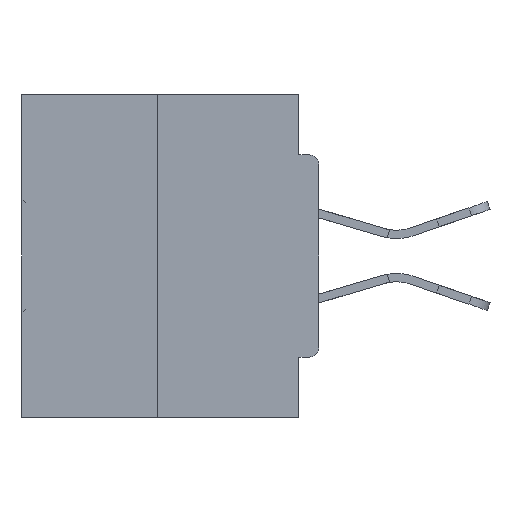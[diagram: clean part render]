
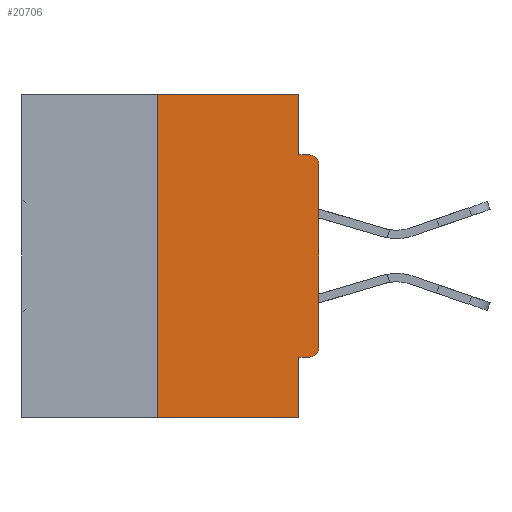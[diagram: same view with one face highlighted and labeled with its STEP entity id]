
A CAD part, left-side view. The second image highlights one B-rep face of the part: STEP entity #20706.
In plain terms, the highlighted planar face has unit normal (-1, 0, 0).
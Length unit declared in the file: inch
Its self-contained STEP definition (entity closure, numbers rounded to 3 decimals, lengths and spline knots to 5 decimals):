
#2132 = CARTESIAN_POINT ( 'NONE',  ( 0., 0.015, -0.3915 ) ) ;
#3215 = ORIENTED_EDGE ( 'NONE', *, *, #10793, .F. ) ;
#3458 = AXIS2_PLACEMENT_3D ( 'NONE', #44078, #10259, #24058 ) ;
#3764 = LINE ( 'NONE', #19741, #40577 ) ;
#4385 = VECTOR ( 'NONE', #37120, 39.37008 ) ;
#5141 = LINE ( 'NONE', #14139, #30230 ) ;
#6019 = EDGE_LOOP ( 'NONE', ( #20802, #9679, #41774, #3215, #23538, #33979, #34503, #25848, #26507, #16166 ) ) ;
#6390 = CARTESIAN_POINT ( 'NONE',  ( 0., 0.25, 0. ) ) ;
#6479 = CARTESIAN_POINT ( 'NONE',  ( 0., 0.015, -0.4065 ) ) ;
#6637 = CARTESIAN_POINT ( 'NONE',  ( 0., 0., 0. ) ) ;
#6655 = PLANE ( 'NONE',  #3458 ) ;
#8766 = EDGE_CURVE ( 'NONE', #9557, #28102, #12929, .T. ) ;
#9229 = EDGE_CURVE ( 'NONE', #41579, #10682, #3764, .T. ) ;
#9557 = VERTEX_POINT ( 'NONE', #23815 ) ;
#9679 = ORIENTED_EDGE ( 'NONE', *, *, #15289, .F. ) ;
#9711 = DIRECTION ( 'NONE',  ( 0., -1., 0. ) ) ;
#10259 = DIRECTION ( 'NONE',  ( 1., 0., 0. ) ) ;
#10342 = VERTEX_POINT ( 'NONE', #38092 ) ;
#10682 = VERTEX_POINT ( 'NONE', #34800 ) ;
#10779 = CARTESIAN_POINT ( 'NONE',  ( 0., 0.46, 0. ) ) ;
#10793 = EDGE_CURVE ( 'NONE', #10682, #10342, #41548, .T. ) ;
#11541 = CARTESIAN_POINT ( 'NONE',  ( 0., 0., -0.3915 ) ) ;
#12639 = DIRECTION ( 'NONE',  ( -1., 0., 0. ) ) ;
#12929 = LINE ( 'NONE', #37290, #25717 ) ;
#13161 = CARTESIAN_POINT ( 'NONE',  ( 0., 0.015, -0.1085 ) ) ;
#13564 = DIRECTION ( 'NONE',  ( 0., 0., 1. ) ) ;
#14139 = CARTESIAN_POINT ( 'NONE',  ( 0., 0.46, -0.5 ) ) ;
#14842 = EDGE_CURVE ( 'NONE', #41579, #28055, #37000, .T. ) ;
#15255 = VECTOR ( 'NONE', #41739, 39.37008 ) ;
#15289 = EDGE_CURVE ( 'NONE', #26956, #26529, #18913, .T. ) ;
#16166 = ORIENTED_EDGE ( 'NONE', *, *, #32819, .F. ) ;
#16823 = AXIS2_PLACEMENT_3D ( 'NONE', #13161, #26415, #23344 ) ;
#18913 = LINE ( 'NONE', #6390, #4385 ) ;
#18950 = DIRECTION ( 'NONE',  ( 0., 0., -1. ) ) ;
#19741 = CARTESIAN_POINT ( 'NONE',  ( 0., 0., -0.4065 ) ) ;
#20706 = ADVANCED_FACE ( 'NONE', ( #24940 ), #6655, .F. ) ;
#20802 = ORIENTED_EDGE ( 'NONE', *, *, #21831, .F. ) ;
#21831 = EDGE_CURVE ( 'NONE', #26529, #32000, #26932, .T. ) ;
#22022 = AXIS2_PLACEMENT_3D ( 'NONE', #2132, #12639, #18950 ) ;
#22962 = LINE ( 'NONE', #6637, #24536 ) ;
#23344 = DIRECTION ( 'NONE',  ( 0., 0., -1. ) ) ;
#23538 = ORIENTED_EDGE ( 'NONE', *, *, #9229, .F. ) ;
#23815 = CARTESIAN_POINT ( 'NONE',  ( 0., 0.031, -0.0935 ) ) ;
#24058 = DIRECTION ( 'NONE',  ( 0., 0., -1. ) ) ;
#24193 = CARTESIAN_POINT ( 'NONE',  ( 0., 0.031, 0. ) ) ;
#24289 = CARTESIAN_POINT ( 'NONE',  ( 0., 0.031, 0. ) ) ;
#24483 = CARTESIAN_POINT ( 'NONE',  ( 0., 0., -0.1085 ) ) ;
#24488 = EDGE_CURVE ( 'NONE', #36658, #28102, #31481, .T. ) ;
#24536 = VECTOR ( 'NONE', #13564, 39.37008 ) ;
#24940 = FACE_OUTER_BOUND ( 'NONE', #6019, .T. ) ;
#25100 = EDGE_CURVE ( 'NONE', #28055, #36658, #22962, .T. ) ;
#25717 = VECTOR ( 'NONE', #9711, 39.37008 ) ;
#25848 = ORIENTED_EDGE ( 'NONE', *, *, #24488, .T. ) ;
#26386 = VECTOR ( 'NONE', #32191, 39.37008 ) ;
#26415 = DIRECTION ( 'NONE',  ( -1., 0., 0. ) ) ;
#26507 = ORIENTED_EDGE ( 'NONE', *, *, #8766, .F. ) ;
#26529 = VERTEX_POINT ( 'NONE', #39012 ) ;
#26932 = LINE ( 'NONE', #10779, #15255 ) ;
#26956 = VERTEX_POINT ( 'NONE', #39835 ) ;
#28055 = VERTEX_POINT ( 'NONE', #11541 ) ;
#28102 = VERTEX_POINT ( 'NONE', #39200 ) ;
#30230 = VECTOR ( 'NONE', #34917, 39.37008 ) ;
#30234 = DIRECTION ( 'NONE',  ( 0., 1., 0. ) ) ;
#31481 = CIRCLE ( 'NONE', #16823, 0.015 ) ;
#32000 = VERTEX_POINT ( 'NONE', #24193 ) ;
#32191 = DIRECTION ( 'NONE',  ( 0., 0., -1. ) ) ;
#32819 = EDGE_CURVE ( 'NONE', #32000, #9557, #35438, .T. ) ;
#33535 = VECTOR ( 'NONE', #44072, 39.37008 ) ;
#33979 = ORIENTED_EDGE ( 'NONE', *, *, #14842, .T. ) ;
#34503 = ORIENTED_EDGE ( 'NONE', *, *, #25100, .T. ) ;
#34800 = CARTESIAN_POINT ( 'NONE',  ( 0., 0.031, -0.4065 ) ) ;
#34917 = DIRECTION ( 'NONE',  ( 0., -1., 0. ) ) ;
#35438 = LINE ( 'NONE', #24289, #26386 ) ;
#35724 = EDGE_CURVE ( 'NONE', #26956, #10342, #5141, .T. ) ;
#36658 = VERTEX_POINT ( 'NONE', #24483 ) ;
#37000 = CIRCLE ( 'NONE', #22022, 0.015 ) ;
#37120 = DIRECTION ( 'NONE',  ( 0., 0., 1. ) ) ;
#37233 = CARTESIAN_POINT ( 'NONE',  ( 0., 0.031, -0.5 ) ) ;
#37290 = CARTESIAN_POINT ( 'NONE',  ( 0., 0., -0.0935 ) ) ;
#38092 = CARTESIAN_POINT ( 'NONE',  ( 0., 0.031, -0.5 ) ) ;
#39012 = CARTESIAN_POINT ( 'NONE',  ( 0., 0.25, 0. ) ) ;
#39200 = CARTESIAN_POINT ( 'NONE',  ( 0., 0.015, -0.0935 ) ) ;
#39835 = CARTESIAN_POINT ( 'NONE',  ( 0., 0.25, -0.5 ) ) ;
#40577 = VECTOR ( 'NONE', #30234, 39.37008 ) ;
#41548 = LINE ( 'NONE', #37233, #33535 ) ;
#41579 = VERTEX_POINT ( 'NONE', #6479 ) ;
#41739 = DIRECTION ( 'NONE',  ( 0., -1., 0. ) ) ;
#41774 = ORIENTED_EDGE ( 'NONE', *, *, #35724, .T. ) ;
#44072 = DIRECTION ( 'NONE',  ( 0., 0., -1. ) ) ;
#44078 = CARTESIAN_POINT ( 'NONE',  ( 0., 0.46, 0. ) ) ;
